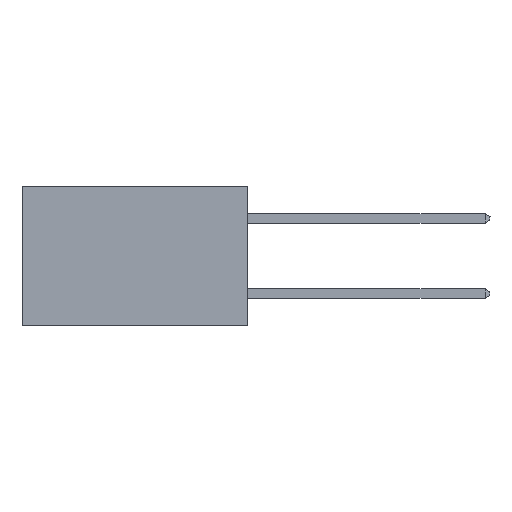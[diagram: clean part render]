
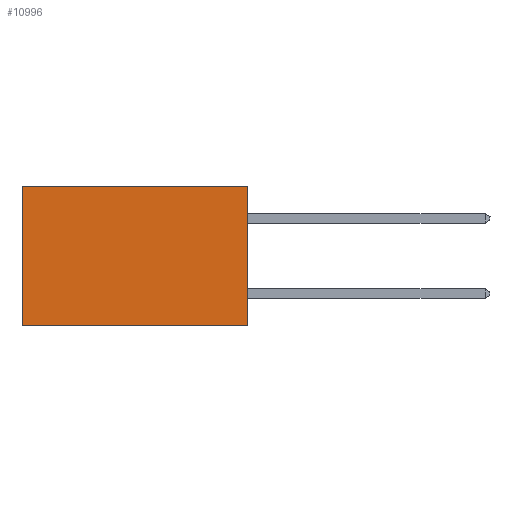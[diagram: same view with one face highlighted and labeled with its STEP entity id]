
A CAD part, left-side view. The second image highlights one B-rep face of the part: STEP entity #10996.
In plain terms, the highlighted planar face has unit normal (-1, 0, 0).
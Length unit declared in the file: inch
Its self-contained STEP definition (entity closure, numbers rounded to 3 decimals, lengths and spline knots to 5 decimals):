
#419 = VERTEX_POINT ( 'NONE', #4310 ) ;
#1066 = AXIS2_PLACEMENT_3D ( 'NONE', #4712, #7374, #9171 ) ;
#1358 = CARTESIAN_POINT ( 'NONE',  ( 0.2615, 0., 0. ) ) ;
#1892 = EDGE_CURVE ( 'NONE', #419, #12698, #2658, .T. ) ;
#2039 = CARTESIAN_POINT ( 'NONE',  ( 0.2615, 0.6, -0.37 ) ) ;
#2040 = VECTOR ( 'NONE', #4513, 39.37008 ) ;
#2120 = VERTEX_POINT ( 'NONE', #6866 ) ;
#2658 = LINE ( 'NONE', #5796, #13383 ) ;
#2938 = CARTESIAN_POINT ( 'NONE',  ( 0.2615, 0., -0.37 ) ) ;
#3554 = DIRECTION ( 'NONE',  ( 0., 1., 0. ) ) ;
#4010 = VERTEX_POINT ( 'NONE', #10725 ) ;
#4264 = ORIENTED_EDGE ( 'NONE', *, *, #13716, .T. ) ;
#4310 = CARTESIAN_POINT ( 'NONE',  ( 0.2615, 0., -0.37 ) ) ;
#4513 = DIRECTION ( 'NONE',  ( 0., 1., 0. ) ) ;
#4545 = EDGE_CURVE ( 'NONE', #4010, #419, #12102, .T. ) ;
#4712 = CARTESIAN_POINT ( 'NONE',  ( 0.2615, 0., -0.37 ) ) ;
#5747 = EDGE_CURVE ( 'NONE', #2120, #12698, #6013, .T. ) ;
#5796 = CARTESIAN_POINT ( 'NONE',  ( 0.2615, 0., -0.37 ) ) ;
#6013 = LINE ( 'NONE', #13965, #8610 ) ;
#6866 = CARTESIAN_POINT ( 'NONE',  ( 0.2615, 0.6, 0. ) ) ;
#7374 = DIRECTION ( 'NONE',  ( 1., 0., 0. ) ) ;
#7757 = ORIENTED_EDGE ( 'NONE', *, *, #1892, .F. ) ;
#7932 = LINE ( 'NONE', #1358, #2040 ) ;
#8602 = ORIENTED_EDGE ( 'NONE', *, *, #4545, .F. ) ;
#8610 = VECTOR ( 'NONE', #13826, 39.37008 ) ;
#9171 = DIRECTION ( 'NONE',  ( 0., 0., -1. ) ) ;
#9204 = ORIENTED_EDGE ( 'NONE', *, *, #5747, .T. ) ;
#9254 = PLANE ( 'NONE',  #1066 ) ;
#9675 = FACE_OUTER_BOUND ( 'NONE', #13675, .T. ) ;
#10725 = CARTESIAN_POINT ( 'NONE',  ( 0.2615, 0., 0. ) ) ;
#10996 = ADVANCED_FACE ( 'NONE', ( #9675 ), #9254, .F. ) ;
#11954 = DIRECTION ( 'NONE',  ( 0., 0., -1. ) ) ;
#12102 = LINE ( 'NONE', #2938, #13717 ) ;
#12698 = VERTEX_POINT ( 'NONE', #2039 ) ;
#13383 = VECTOR ( 'NONE', #3554, 39.37008 ) ;
#13675 = EDGE_LOOP ( 'NONE', ( #9204, #7757, #8602, #4264 ) ) ;
#13716 = EDGE_CURVE ( 'NONE', #4010, #2120, #7932, .T. ) ;
#13717 = VECTOR ( 'NONE', #11954, 39.37008 ) ;
#13826 = DIRECTION ( 'NONE',  ( 0., 0., -1. ) ) ;
#13965 = CARTESIAN_POINT ( 'NONE',  ( 0.2615, 0.6, -0.37 ) ) ;
